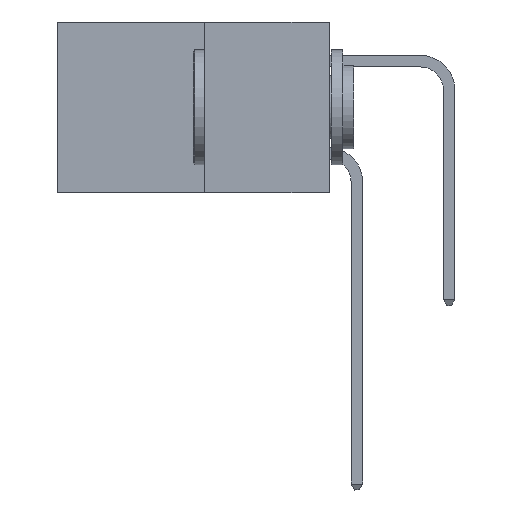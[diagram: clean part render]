
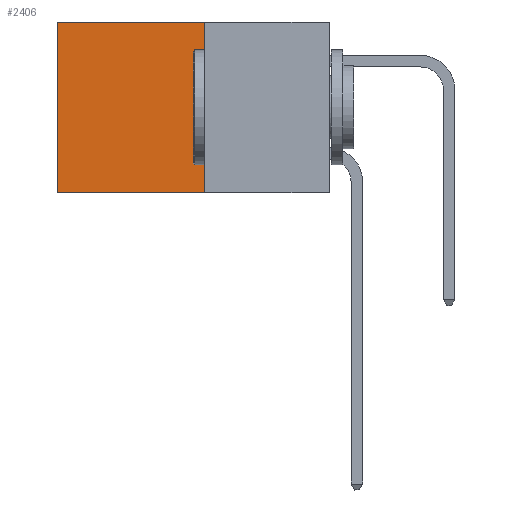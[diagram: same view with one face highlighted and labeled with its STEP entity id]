
A CAD part, left-side view. The second image highlights one B-rep face of the part: STEP entity #2406.
In plain terms, the highlighted planar face has unit normal (-1, 0, 0).
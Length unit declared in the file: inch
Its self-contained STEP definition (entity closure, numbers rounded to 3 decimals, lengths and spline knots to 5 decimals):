
#365 = LINE ( 'NONE', #7115, #7255 ) ;
#749 = EDGE_CURVE ( 'NONE', #4440, #8245, #365, .T. ) ;
#1053 = DIRECTION ( 'NONE',  ( 0., 1., 0. ) ) ;
#1198 = VECTOR ( 'NONE', #10895, 39.37008 ) ;
#1479 = VERTEX_POINT ( 'NONE', #4016 ) ;
#2063 = PLANE ( 'NONE',  #9322 ) ;
#2089 = VECTOR ( 'NONE', #2717, 39.37008 ) ;
#2119 = DIRECTION ( 'NONE',  ( 1., 0., 0. ) ) ;
#2406 = ADVANCED_FACE ( 'NONE', ( #2575 ), #2063, .F. ) ;
#2575 = FACE_OUTER_BOUND ( 'NONE', #10236, .T. ) ;
#2717 = DIRECTION ( 'NONE',  ( 0., 0., -1. ) ) ;
#2728 = CARTESIAN_POINT ( 'NONE',  ( 0.277, 0.59, 0. ) ) ;
#3187 = CARTESIAN_POINT ( 'NONE',  ( 0.277, 0.27, -0.37 ) ) ;
#3278 = CARTESIAN_POINT ( 'NONE',  ( 0.277, 0.27, 0. ) ) ;
#3940 = EDGE_CURVE ( 'NONE', #8245, #11074, #4488, .T. ) ;
#4016 = CARTESIAN_POINT ( 'NONE',  ( 0.277, 0.27, -0.37 ) ) ;
#4229 = DIRECTION ( 'NONE',  ( 0., 0., -1. ) ) ;
#4440 = VERTEX_POINT ( 'NONE', #3278 ) ;
#4488 = LINE ( 'NONE', #7907, #2089 ) ;
#5288 = ORIENTED_EDGE ( 'NONE', *, *, #3940, .T. ) ;
#5492 = CARTESIAN_POINT ( 'NONE',  ( 0.277, 0.59, -0.37 ) ) ;
#5571 = ORIENTED_EDGE ( 'NONE', *, *, #749, .T. ) ;
#5619 = DIRECTION ( 'NONE',  ( 0., 0., -1. ) ) ;
#6212 = LINE ( 'NONE', #6699, #1198 ) ;
#6699 = CARTESIAN_POINT ( 'NONE',  ( 0.277, 0.27, -0.37 ) ) ;
#6754 = LINE ( 'NONE', #9833, #10957 ) ;
#7115 = CARTESIAN_POINT ( 'NONE',  ( 0.277, 0.27, 0. ) ) ;
#7255 = VECTOR ( 'NONE', #1053, 39.37008 ) ;
#7591 = ORIENTED_EDGE ( 'NONE', *, *, #9451, .F. ) ;
#7907 = CARTESIAN_POINT ( 'NONE',  ( 0.277, 0.59, -0.37 ) ) ;
#8245 = VERTEX_POINT ( 'NONE', #2728 ) ;
#8494 = EDGE_CURVE ( 'NONE', #4440, #1479, #6754, .T. ) ;
#9322 = AXIS2_PLACEMENT_3D ( 'NONE', #3187, #2119, #4229 ) ;
#9451 = EDGE_CURVE ( 'NONE', #1479, #11074, #6212, .T. ) ;
#9803 = ORIENTED_EDGE ( 'NONE', *, *, #8494, .F. ) ;
#9833 = CARTESIAN_POINT ( 'NONE',  ( 0.277, 0.27, -0.37 ) ) ;
#10236 = EDGE_LOOP ( 'NONE', ( #5288, #7591, #9803, #5571 ) ) ;
#10895 = DIRECTION ( 'NONE',  ( 0., 1., 0. ) ) ;
#10957 = VECTOR ( 'NONE', #5619, 39.37008 ) ;
#11074 = VERTEX_POINT ( 'NONE', #5492 ) ;
